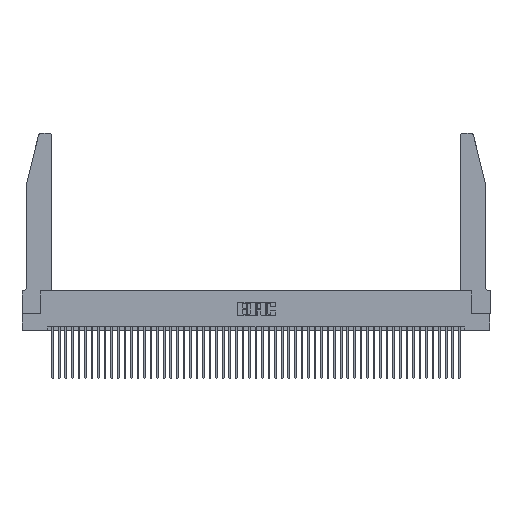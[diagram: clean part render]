
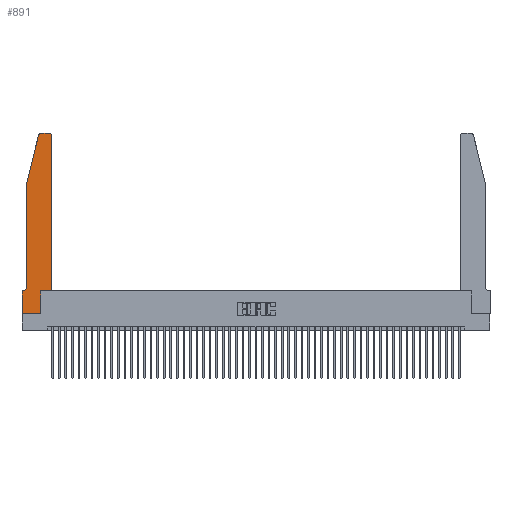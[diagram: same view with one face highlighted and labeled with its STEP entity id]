
A CAD part, top view. The second image highlights one B-rep face of the part: STEP entity #891.
In plain terms, the highlighted planar face has unit normal (0, 0, 1).
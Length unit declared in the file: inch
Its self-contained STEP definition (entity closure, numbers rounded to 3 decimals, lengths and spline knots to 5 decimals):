
#313 = VERTEX_POINT ( 'NONE', #15187 ) ;
#891 = ADVANCED_FACE ( 'NONE', ( #37468 ), #46987, .T. ) ;
#1271 = EDGE_CURVE ( 'NONE', #9039, #8900, #10671, .T. ) ;
#1298 = CARTESIAN_POINT ( 'NONE',  ( 0.0755, 2., 0.37 ) ) ;
#1421 = CARTESIAN_POINT ( 'NONE',  ( 0.4505, 0.35, 0.37 ) ) ;
#1780 = DIRECTION ( 'NONE',  ( 1., 0., 0. ) ) ;
#2059 = CARTESIAN_POINT ( 'NONE',  ( 0.0755, 2., 0.37 ) ) ;
#2626 = DIRECTION ( 'NONE',  ( 0., 0., -1. ) ) ;
#2926 = VERTEX_POINT ( 'NONE', #8797 ) ;
#2958 = ORIENTED_EDGE ( 'NONE', *, *, #33594, .T. ) ;
#3025 = VECTOR ( 'NONE', #49600, 39.37008 ) ;
#3809 = EDGE_CURVE ( 'NONE', #48325, #9039, #30870, .T. ) ;
#4570 = ORIENTED_EDGE ( 'NONE', *, *, #23009, .T. ) ;
#5506 = DIRECTION ( 'NONE',  ( 0., 0., 1. ) ) ;
#5734 = EDGE_CURVE ( 'NONE', #47114, #40583, #42368, .T. ) ;
#5897 = EDGE_CURVE ( 'NONE', #6773, #12274, #33748, .T. ) ;
#6454 = DIRECTION ( 'NONE',  ( 0., 1., 0. ) ) ;
#6773 = VERTEX_POINT ( 'NONE', #27476 ) ;
#7259 = CARTESIAN_POINT ( 'NONE',  ( 0., 0.35, 0.37 ) ) ;
#8797 = CARTESIAN_POINT ( 'NONE',  ( 0.4205, 2.75, 0.37 ) ) ;
#8900 = VERTEX_POINT ( 'NONE', #40303 ) ;
#9039 = VERTEX_POINT ( 'NONE', #14916 ) ;
#9174 = CARTESIAN_POINT ( 'NONE',  ( 0.2605, 2.75, 0.37 ) ) ;
#9596 = DIRECTION ( 'NONE',  ( 0., 0., 1. ) ) ;
#9905 = ORIENTED_EDGE ( 'NONE', *, *, #5897, .T. ) ;
#10445 = LINE ( 'NONE', #32536, #51286 ) ;
#10671 = LINE ( 'NONE', #1421, #21311 ) ;
#11481 = ORIENTED_EDGE ( 'NONE', *, *, #35672, .T. ) ;
#12238 = EDGE_CURVE ( 'NONE', #8900, #15746, #10445, .T. ) ;
#12274 = VERTEX_POINT ( 'NONE', #32885 ) ;
#14916 = CARTESIAN_POINT ( 'NONE',  ( 0.2865, 0.35, 0.37 ) ) ;
#15187 = CARTESIAN_POINT ( 'NONE',  ( 0.284, 2.75, 0.37 ) ) ;
#15746 = VERTEX_POINT ( 'NONE', #37597 ) ;
#16717 = DIRECTION ( 'NONE',  ( 0., 1., 0. ) ) ;
#18229 = EDGE_CURVE ( 'NONE', #2926, #313, #19535, .T. ) ;
#18536 = CARTESIAN_POINT ( 'NONE',  ( 0.2865, 0.35, 0.37 ) ) ;
#19535 = LINE ( 'NONE', #9174, #49787 ) ;
#19885 = EDGE_CURVE ( 'NONE', #15746, #2926, #37365, .T. ) ;
#20502 = LINE ( 'NONE', #35835, #40332 ) ;
#20990 = ORIENTED_EDGE ( 'NONE', *, *, #19885, .T. ) ;
#21311 = VECTOR ( 'NONE', #33393, 39.37008 ) ;
#21587 = VECTOR ( 'NONE', #6454, 39.37008 ) ;
#21912 = AXIS2_PLACEMENT_3D ( 'NONE', #33486, #9596, #37438 ) ;
#21941 = VECTOR ( 'NONE', #34500, 39.37008 ) ;
#22541 = CARTESIAN_POINT ( 'NONE',  ( 0., 0., 0.37 ) ) ;
#23009 = EDGE_CURVE ( 'NONE', #49970, #47114, #24208, .T. ) ;
#23346 = DIRECTION ( 'NONE',  ( 0., 0., 1. ) ) ;
#24005 = AXIS2_PLACEMENT_3D ( 'NONE', #7259, #23346, #50895 ) ;
#24208 = LINE ( 'NONE', #1298, #25466 ) ;
#24893 = ORIENTED_EDGE ( 'NONE', *, *, #43457, .T. ) ;
#25355 = EDGE_LOOP ( 'NONE', ( #40060, #11481, #4570, #26104, #2958, #24893, #9905, #35220, #40184, #39585, #28393, #20990 ) ) ;
#25385 = VERTEX_POINT ( 'NONE', #28054 ) ;
#25466 = VECTOR ( 'NONE', #27999, 39.37008 ) ;
#26104 = ORIENTED_EDGE ( 'NONE', *, *, #5734, .T. ) ;
#26583 = CARTESIAN_POINT ( 'NONE',  ( 0.0055, 0.42, 0.37 ) ) ;
#27476 = CARTESIAN_POINT ( 'NONE',  ( 0., 0.35, 0.37 ) ) ;
#27999 = DIRECTION ( 'NONE',  ( -0.239, -0.971, 0. ) ) ;
#28054 = CARTESIAN_POINT ( 'NONE',  ( 0.0055, 0.35, 0.37 ) ) ;
#28393 = ORIENTED_EDGE ( 'NONE', *, *, #12238, .T. ) ;
#29040 = CARTESIAN_POINT ( 'NONE',  ( 0.0755, 2., 0.37 ) ) ;
#29431 = CARTESIAN_POINT ( 'NONE',  ( 0.4205, 2.72, 0.37 ) ) ;
#29730 = CARTESIAN_POINT ( 'NONE',  ( 0., 0., 0.37 ) ) ;
#30540 = DIRECTION ( 'NONE',  ( -1., 0., 0. ) ) ;
#30870 = LINE ( 'NONE', #18536, #21587 ) ;
#32536 = CARTESIAN_POINT ( 'NONE',  ( 0.4505, 0.35, 0.37 ) ) ;
#32885 = CARTESIAN_POINT ( 'NONE',  ( 0., 0., 0.37 ) ) ;
#33393 = DIRECTION ( 'NONE',  ( 1., 0., 0. ) ) ;
#33436 = DIRECTION ( 'NONE',  ( 1., 0., 0. ) ) ;
#33486 = CARTESIAN_POINT ( 'NONE',  ( 0.284, 2.72, 0.37 ) ) ;
#33594 = EDGE_CURVE ( 'NONE', #40583, #25385, #39285, .T. ) ;
#33748 = LINE ( 'NONE', #22541, #21941 ) ;
#34500 = DIRECTION ( 'NONE',  ( 0., -1., 0. ) ) ;
#34913 = LINE ( 'NONE', #29730, #44134 ) ;
#35220 = ORIENTED_EDGE ( 'NONE', *, *, #41342, .T. ) ;
#35672 = EDGE_CURVE ( 'NONE', #313, #49970, #42046, .T. ) ;
#35821 = AXIS2_PLACEMENT_3D ( 'NONE', #26583, #2626, #30540 ) ;
#35835 = CARTESIAN_POINT ( 'NONE',  ( 0.0755, 0.35, 0.37 ) ) ;
#36579 = CARTESIAN_POINT ( 'NONE',  ( 0.0755, 0.42, 0.37 ) ) ;
#37041 = DIRECTION ( 'NONE',  ( -1., 0., 0. ) ) ;
#37365 = CIRCLE ( 'NONE', #39066, 0.03 ) ;
#37438 = DIRECTION ( 'NONE',  ( 1., 0., 0. ) ) ;
#37468 = FACE_OUTER_BOUND ( 'NONE', #25355, .T. ) ;
#37597 = CARTESIAN_POINT ( 'NONE',  ( 0.4505, 2.72, 0.37 ) ) ;
#37806 = CARTESIAN_POINT ( 'NONE',  ( 0.25487, 2.72718, 0.37 ) ) ;
#39066 = AXIS2_PLACEMENT_3D ( 'NONE', #29431, #5506, #33436 ) ;
#39285 = CIRCLE ( 'NONE', #35821, 0.07 ) ;
#39585 = ORIENTED_EDGE ( 'NONE', *, *, #1271, .T. ) ;
#40060 = ORIENTED_EDGE ( 'NONE', *, *, #18229, .T. ) ;
#40184 = ORIENTED_EDGE ( 'NONE', *, *, #3809, .T. ) ;
#40303 = CARTESIAN_POINT ( 'NONE',  ( 0.4505, 0.35, 0.37 ) ) ;
#40332 = VECTOR ( 'NONE', #43549, 39.37008 ) ;
#40583 = VERTEX_POINT ( 'NONE', #36579 ) ;
#41342 = EDGE_CURVE ( 'NONE', #12274, #48325, #34913, .T. ) ;
#42046 = CIRCLE ( 'NONE', #21912, 0.03 ) ;
#42368 = LINE ( 'NONE', #2059, #3025 ) ;
#43246 = CARTESIAN_POINT ( 'NONE',  ( 0.2865, 0., 0.37 ) ) ;
#43457 = EDGE_CURVE ( 'NONE', #25385, #6773, #20502, .T. ) ;
#43549 = DIRECTION ( 'NONE',  ( -1., 0., 0. ) ) ;
#44134 = VECTOR ( 'NONE', #1780, 39.37008 ) ;
#46987 = PLANE ( 'NONE',  #24005 ) ;
#47114 = VERTEX_POINT ( 'NONE', #29040 ) ;
#48325 = VERTEX_POINT ( 'NONE', #43246 ) ;
#49600 = DIRECTION ( 'NONE',  ( 0., -1., 0. ) ) ;
#49787 = VECTOR ( 'NONE', #37041, 39.37008 ) ;
#49970 = VERTEX_POINT ( 'NONE', #37806 ) ;
#50895 = DIRECTION ( 'NONE',  ( 1., 0., 0. ) ) ;
#51286 = VECTOR ( 'NONE', #16717, 39.37008 ) ;
